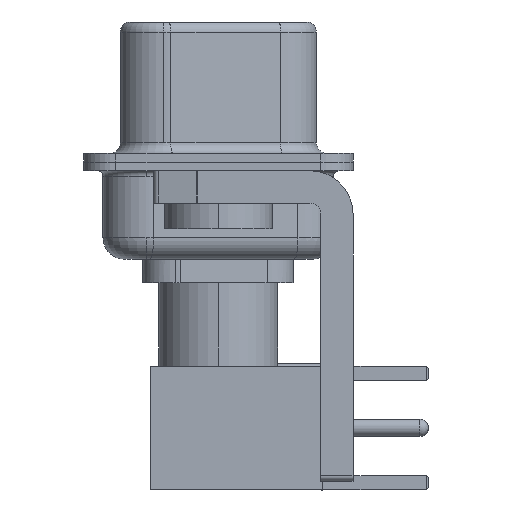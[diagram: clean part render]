
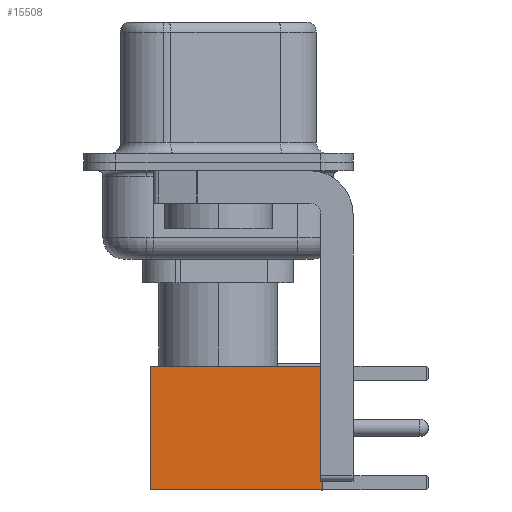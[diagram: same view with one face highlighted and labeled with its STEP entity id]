
A CAD part, left-side view. The second image highlights one B-rep face of the part: STEP entity #15508.
In plain terms, the highlighted face is planar.
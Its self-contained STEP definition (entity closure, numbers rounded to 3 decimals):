
#538 = AXIS2_PLACEMENT_3D ( 'NONE', #13136, #1112, #13754 ) ;
#892 = CARTESIAN_POINT ( 'NONE',  ( 0., 2.875, 0. ) ) ;
#928 = DIRECTION ( 'NONE',  ( -1., 0., 0. ) ) ;
#1112 = DIRECTION ( 'NONE',  ( 0., 1., 0. ) ) ;
#1974 = EDGE_CURVE ( 'NONE', #2174, #17826, #13795, .T. ) ;
#2174 = VERTEX_POINT ( 'NONE', #24602 ) ;
#2976 = ORIENTED_EDGE ( 'NONE', *, *, #21989, .T. ) ;
#4423 = ORIENTED_EDGE ( 'NONE', *, *, #1974, .T. ) ;
#6556 = CARTESIAN_POINT ( 'NONE',  ( -2.875, 2.875, 0. ) ) ;
#6600 = VECTOR ( 'NONE', #6912, 1000. ) ;
#6912 = DIRECTION ( 'NONE',  ( 0., 0., -1. ) ) ;
#8566 = CARTESIAN_POINT ( 'NONE',  ( 0., 2.875, 8. ) ) ;
#11591 = EDGE_CURVE ( 'NONE', #24254, #15405, #28838, .T. ) ;
#11693 = ORIENTED_EDGE ( 'NONE', *, *, #13559, .F. ) ;
#12209 = CARTESIAN_POINT ( 'NONE',  ( -2.875, 2.875, 0. ) ) ;
#12984 = PLANE ( 'NONE',  #538 ) ;
#13136 = CARTESIAN_POINT ( 'NONE',  ( 2.875, 2.875, 0. ) ) ;
#13559 = EDGE_CURVE ( 'NONE', #2174, #24254, #25027, .T. ) ;
#13642 = VECTOR ( 'NONE', #928, 1000. ) ;
#13743 = VECTOR ( 'NONE', #21291, 1000. ) ;
#13754 = DIRECTION ( 'NONE',  ( 0., 0., 1. ) ) ;
#13795 = LINE ( 'NONE', #14247, #6600 ) ;
#14057 = LINE ( 'NONE', #892, #13743 ) ;
#14247 = CARTESIAN_POINT ( 'NONE',  ( 2.875, 2.875, 0. ) ) ;
#15405 = VERTEX_POINT ( 'NONE', #6556 ) ;
#15508 = ADVANCED_FACE ( 'NONE', ( #16116 ), #12984, .T. ) ;
#16116 = FACE_OUTER_BOUND ( 'NONE', #30104, .T. ) ;
#16904 = DIRECTION ( 'NONE',  ( 0., 0., -1. ) ) ;
#17637 = ORIENTED_EDGE ( 'NONE', *, *, #11591, .F. ) ;
#17826 = VERTEX_POINT ( 'NONE', #27206 ) ;
#17870 = VECTOR ( 'NONE', #16904, 1000. ) ;
#21291 = DIRECTION ( 'NONE',  ( -1., 0., 0. ) ) ;
#21989 = EDGE_CURVE ( 'NONE', #17826, #15405, #14057, .T. ) ;
#24254 = VERTEX_POINT ( 'NONE', #27781 ) ;
#24602 = CARTESIAN_POINT ( 'NONE',  ( 2.875, 2.875, 8. ) ) ;
#25027 = LINE ( 'NONE', #8566, #13642 ) ;
#27206 = CARTESIAN_POINT ( 'NONE',  ( 2.875, 2.875, 0. ) ) ;
#27781 = CARTESIAN_POINT ( 'NONE',  ( -2.875, 2.875, 8. ) ) ;
#28838 = LINE ( 'NONE', #12209, #17870 ) ;
#30104 = EDGE_LOOP ( 'NONE', ( #4423, #2976, #17637, #11693 ) ) ;
